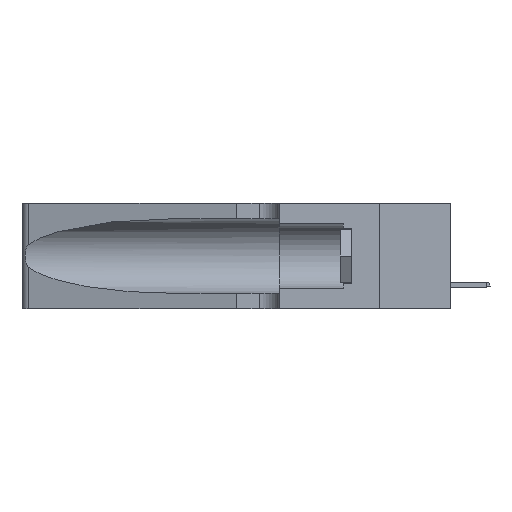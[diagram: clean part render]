
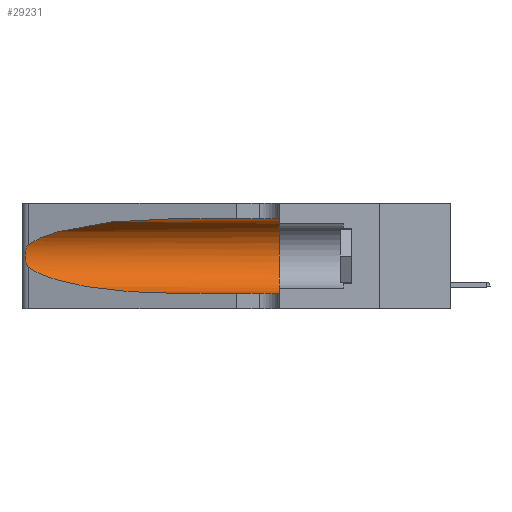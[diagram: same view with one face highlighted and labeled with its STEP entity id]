
A CAD part, left-side view. The second image highlights one B-rep face of the part: STEP entity #29231.
In plain terms, the highlighted cylindrical face has radius 3.308 mm (diameter 6.617 mm), a partial arc.
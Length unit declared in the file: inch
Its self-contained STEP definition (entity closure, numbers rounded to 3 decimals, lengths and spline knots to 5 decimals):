
#379 = CARTESIAN_POINT ( 'NONE',  ( 0.25639, 1.23186, 0.15144 ) ) ;
#422 = AXIS2_PLACEMENT_3D ( 'NONE', #18433, #9843, #4705 ) ;
#1404 = CARTESIAN_POINT ( 'NONE',  ( 0.18966, 0.96281, 0.31525 ) ) ;
#1810 = CARTESIAN_POINT ( 'NONE',  ( 0.25487, 1.22718, 0.14631 ) ) ;
#2022 = CARTESIAN_POINT ( 'NONE',  ( 0.1305, 0.35, 0.31525 ) ) ;
#2276 = VERTEX_POINT ( 'NONE', #29047 ) ;
#3448 = AXIS2_PLACEMENT_3D ( 'NONE', #5284, #27683, #18487 ) ;
#3644 = B_SPLINE_CURVE_WITH_KNOTS ( 'NONE', 3,
 ( #29811, #5008, #23941, #4484, #10699, #21887, #33105, #7935, #11244, #28129, #25372, #379, #22433, #22790 ),
 .UNSPECIFIED., .F., .F.,
 ( 4, 2, 2, 2, 2, 2, 4 ),
 ( 0., 0.00027, 0.00053, 0.00107, 0.0016, 0.00187, 0.00214 ),
 .UNSPECIFIED. ) ;
#3978 = CARTESIAN_POINT ( 'NONE',  ( 0.25487, 1.22718, 0.22369 ) ) ;
#4484 = CARTESIAN_POINT ( 'NONE',  ( 0.25787, 1.23484, 0.2124 ) ) ;
#4705 = DIRECTION ( 'NONE',  ( 0., 0., -1. ) ) ;
#5008 = CARTESIAN_POINT ( 'NONE',  ( 0.25555, 1.22994, 0.2215 ) ) ;
#5263 = EDGE_CURVE ( 'NONE', #23454, #9833, #12643, .T. ) ;
#5284 = CARTESIAN_POINT ( 'NONE',  ( 0.1305, 0.35, 0.185 ) ) ;
#5381 = EDGE_CURVE ( 'NONE', #33702, #9833, #21642, .T. ) ;
#6225 =( BOUNDED_CURVE ( )  B_SPLINE_CURVE ( 3, ( #12433, #1404, #17731, #3978 ),
 .UNSPECIFIED., .F., .F. ) 
 B_SPLINE_CURVE_WITH_KNOTS ( ( 4, 4 ),
 ( 1.5708, 2.84003 ),
 .UNSPECIFIED. ) 
 CURVE ( )  GEOMETRIC_REPRESENTATION_ITEM ( )  RATIONAL_B_SPLINE_CURVE ( ( 1., 0.87, 0.87, 1. ) ) 
 REPRESENTATION_ITEM ( '' )  );
#6387 = EDGE_CURVE ( 'NONE', #2276, #23454, #10940, .T. ) ;
#7334 = CARTESIAN_POINT ( 'NONE',  ( 0.18966, 0.96281, 0.05475 ) ) ;
#7583 = EDGE_CURVE ( 'NONE', #25037, #21866, #6225, .T. ) ;
#7935 = CARTESIAN_POINT ( 'NONE',  ( 0.26075, 1.23896, 0.178 ) ) ;
#9405 = CARTESIAN_POINT ( 'NONE',  ( 0.1305, 0.72297, 0.31525 ) ) ;
#9833 = VERTEX_POINT ( 'NONE', #11793 ) ;
#9843 = DIRECTION ( 'NONE',  ( 0., -1., 0. ) ) ;
#10699 = CARTESIAN_POINT ( 'NONE',  ( 0.25854, 1.2359, 0.20912 ) ) ;
#10710 = ORIENTED_EDGE ( 'NONE', *, *, #12403, .F. ) ;
#10940 =( BOUNDED_CURVE ( )  B_SPLINE_CURVE ( 3, ( #1810, #23679, #7334, #26435 ),
 .UNSPECIFIED., .F., .F. ) 
 B_SPLINE_CURVE_WITH_KNOTS ( ( 4, 4 ),
 ( 3.44316, 4.71239 ),
 .UNSPECIFIED. ) 
 CURVE ( )  GEOMETRIC_REPRESENTATION_ITEM ( )  RATIONAL_B_SPLINE_CURVE ( ( 1., 0.87, 0.87, 1. ) ) 
 REPRESENTATION_ITEM ( '' )  );
#11168 = ORIENTED_EDGE ( 'NONE', *, *, #33401, .T. ) ;
#11244 = CARTESIAN_POINT ( 'NONE',  ( 0.26017, 1.23833, 0.17102 ) ) ;
#11793 = CARTESIAN_POINT ( 'NONE',  ( 0.1305, 0.35, 0.05475 ) ) ;
#12403 = EDGE_CURVE ( 'NONE', #25037, #33702, #22675, .T. ) ;
#12433 = CARTESIAN_POINT ( 'NONE',  ( 0.1305, 0.72297, 0.31525 ) ) ;
#12643 = LINE ( 'NONE', #15580, #35144 ) ;
#13679 = EDGE_LOOP ( 'NONE', ( #24685, #11168, #14571, #15560, #25225, #10710 ) ) ;
#14571 = ORIENTED_EDGE ( 'NONE', *, *, #6387, .T. ) ;
#15560 = ORIENTED_EDGE ( 'NONE', *, *, #5263, .T. ) ;
#15580 = CARTESIAN_POINT ( 'NONE',  ( 0.1305, 1.61858, 0.05475 ) ) ;
#17581 = DIRECTION ( 'NONE',  ( 0., -1., 0. ) ) ;
#17731 = CARTESIAN_POINT ( 'NONE',  ( 0.2373, 1.15595, 0.28018 ) ) ;
#18433 = CARTESIAN_POINT ( 'NONE',  ( 0.1305, 1.61858, 0.185 ) ) ;
#18487 = DIRECTION ( 'NONE',  ( 0., 0., 1. ) ) ;
#18796 = CYLINDRICAL_SURFACE ( 'NONE', #422, 0.13025 ) ;
#21642 = CIRCLE ( 'NONE', #3448, 0.13025 ) ;
#21866 = VERTEX_POINT ( 'NONE', #23223 ) ;
#21887 = CARTESIAN_POINT ( 'NONE',  ( 0.26018, 1.23835, 0.19895 ) ) ;
#22433 = CARTESIAN_POINT ( 'NONE',  ( 0.25555, 1.22993, 0.14849 ) ) ;
#22675 = LINE ( 'NONE', #31489, #24543 ) ;
#22790 = CARTESIAN_POINT ( 'NONE',  ( 0.25487, 1.22718, 0.14631 ) ) ;
#23015 = CARTESIAN_POINT ( 'NONE',  ( 0.1305, 0.72297, 0.05475 ) ) ;
#23223 = CARTESIAN_POINT ( 'NONE',  ( 0.25487, 1.22718, 0.22369 ) ) ;
#23454 = VERTEX_POINT ( 'NONE', #23015 ) ;
#23679 = CARTESIAN_POINT ( 'NONE',  ( 0.2373, 1.15595, 0.08982 ) ) ;
#23941 = CARTESIAN_POINT ( 'NONE',  ( 0.25639, 1.23184, 0.21858 ) ) ;
#24543 = VECTOR ( 'NONE', #28212, 39.37008 ) ;
#24685 = ORIENTED_EDGE ( 'NONE', *, *, #7583, .T. ) ;
#25037 = VERTEX_POINT ( 'NONE', #9405 ) ;
#25225 = ORIENTED_EDGE ( 'NONE', *, *, #5381, .F. ) ;
#25372 = CARTESIAN_POINT ( 'NONE',  ( 0.25789, 1.23486, 0.15765 ) ) ;
#26435 = CARTESIAN_POINT ( 'NONE',  ( 0.1305, 0.72297, 0.05475 ) ) ;
#27683 = DIRECTION ( 'NONE',  ( 0., 1., 0. ) ) ;
#28129 = CARTESIAN_POINT ( 'NONE',  ( 0.25856, 1.23593, 0.16098 ) ) ;
#28212 = DIRECTION ( 'NONE',  ( 0., -1., 0. ) ) ;
#29047 = CARTESIAN_POINT ( 'NONE',  ( 0.25487, 1.22718, 0.14631 ) ) ;
#29231 = ADVANCED_FACE ( 'NONE', ( #34833 ), #18796, .F. ) ;
#29811 = CARTESIAN_POINT ( 'NONE',  ( 0.25487, 1.22718, 0.22369 ) ) ;
#31489 = CARTESIAN_POINT ( 'NONE',  ( 0.1305, 1.61858, 0.31525 ) ) ;
#33105 = CARTESIAN_POINT ( 'NONE',  ( 0.26075, 1.23896, 0.19203 ) ) ;
#33401 = EDGE_CURVE ( 'NONE', #21866, #2276, #3644, .T. ) ;
#33702 = VERTEX_POINT ( 'NONE', #2022 ) ;
#34833 = FACE_OUTER_BOUND ( 'NONE', #13679, .T. ) ;
#35144 = VECTOR ( 'NONE', #17581, 39.37008 ) ;
